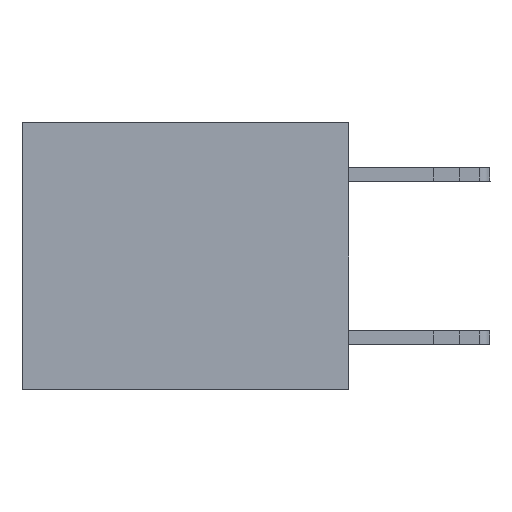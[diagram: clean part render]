
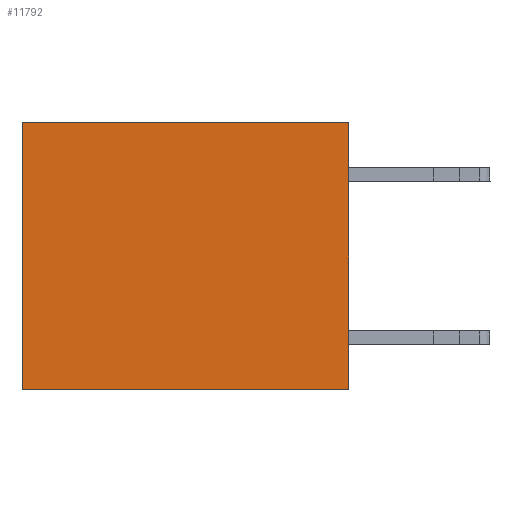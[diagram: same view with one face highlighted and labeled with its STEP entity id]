
A CAD part, left-side view. The second image highlights one B-rep face of the part: STEP entity #11792.
In plain terms, the highlighted planar face has unit normal (-1, 0, 0).
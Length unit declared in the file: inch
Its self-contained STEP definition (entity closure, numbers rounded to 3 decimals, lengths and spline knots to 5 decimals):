
#2185 = CARTESIAN_POINT ( 'NONE',  ( 0.3165, 0.6, -0.49 ) ) ;
#3068 = CARTESIAN_POINT ( 'NONE',  ( 0.3165, 0., -0.49 ) ) ;
#3140 = CARTESIAN_POINT ( 'NONE',  ( 0.3165, 0., 0. ) ) ;
#4037 = VERTEX_POINT ( 'NONE', #22501 ) ;
#6495 = ORIENTED_EDGE ( 'NONE', *, *, #16218, .F. ) ;
#6897 = AXIS2_PLACEMENT_3D ( 'NONE', #26483, #28945, #24277 ) ;
#6974 = LINE ( 'NONE', #20666, #28508 ) ;
#8512 = EDGE_CURVE ( 'NONE', #4037, #15084, #18349, .T. ) ;
#8689 = DIRECTION ( 'NONE',  ( 0., 1., 0. ) ) ;
#9495 = CARTESIAN_POINT ( 'NONE',  ( 0.3165, 0.6, 0. ) ) ;
#9604 = VERTEX_POINT ( 'NONE', #20455 ) ;
#10879 = VERTEX_POINT ( 'NONE', #19315 ) ;
#11792 = ADVANCED_FACE ( 'NONE', ( #18909 ), #14658, .F. ) ;
#13383 = VECTOR ( 'NONE', #16586, 39.37008 ) ;
#14658 = PLANE ( 'NONE',  #6897 ) ;
#15084 = VERTEX_POINT ( 'NONE', #9495 ) ;
#15547 = ORIENTED_EDGE ( 'NONE', *, *, #31046, .T. ) ;
#16218 = EDGE_CURVE ( 'NONE', #9604, #10879, #6974, .T. ) ;
#16311 = VECTOR ( 'NONE', #19927, 39.37008 ) ;
#16586 = DIRECTION ( 'NONE',  ( 0., 0., -1. ) ) ;
#16702 = LINE ( 'NONE', #3068, #16311 ) ;
#17275 = DIRECTION ( 'NONE',  ( 0., 1., 0. ) ) ;
#18349 = LINE ( 'NONE', #3140, #21331 ) ;
#18909 = FACE_OUTER_BOUND ( 'NONE', #28235, .T. ) ;
#19315 = CARTESIAN_POINT ( 'NONE',  ( 0.3165, 0.6, -0.49 ) ) ;
#19927 = DIRECTION ( 'NONE',  ( 0., 0., -1. ) ) ;
#20455 = CARTESIAN_POINT ( 'NONE',  ( 0.3165, 0., -0.49 ) ) ;
#20666 = CARTESIAN_POINT ( 'NONE',  ( 0.3165, 0., -0.49 ) ) ;
#21331 = VECTOR ( 'NONE', #17275, 39.37008 ) ;
#22501 = CARTESIAN_POINT ( 'NONE',  ( 0.3165, 0., 0. ) ) ;
#23768 = ORIENTED_EDGE ( 'NONE', *, *, #8512, .T. ) ;
#24277 = DIRECTION ( 'NONE',  ( 0., 0., -1. ) ) ;
#26483 = CARTESIAN_POINT ( 'NONE',  ( 0.3165, 0., -0.49 ) ) ;
#26510 = EDGE_CURVE ( 'NONE', #4037, #9604, #16702, .T. ) ;
#28235 = EDGE_LOOP ( 'NONE', ( #15547, #6495, #28892, #23768 ) ) ;
#28508 = VECTOR ( 'NONE', #8689, 39.37008 ) ;
#28892 = ORIENTED_EDGE ( 'NONE', *, *, #26510, .F. ) ;
#28945 = DIRECTION ( 'NONE',  ( 1., 0., 0. ) ) ;
#30072 = LINE ( 'NONE', #2185, #13383 ) ;
#31046 = EDGE_CURVE ( 'NONE', #15084, #10879, #30072, .T. ) ;
